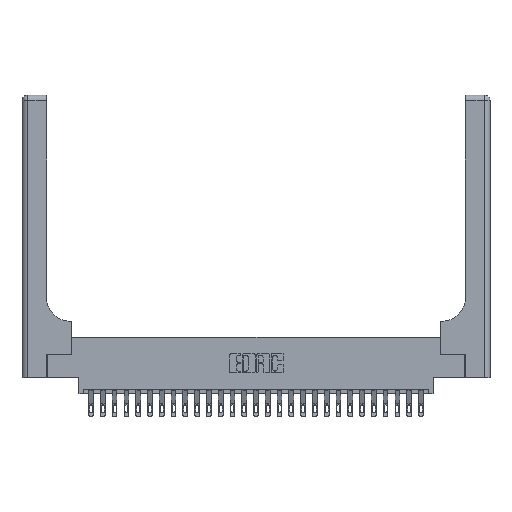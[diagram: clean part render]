
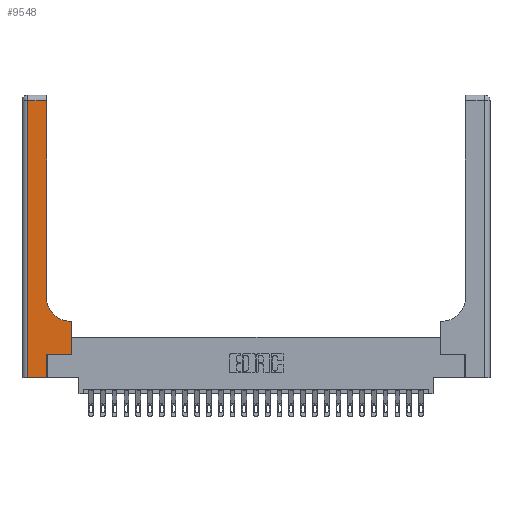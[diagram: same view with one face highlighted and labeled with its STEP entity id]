
A CAD part, top view. The second image highlights one B-rep face of the part: STEP entity #9548.
In plain terms, the highlighted planar face has unit normal (0, 0, 1).
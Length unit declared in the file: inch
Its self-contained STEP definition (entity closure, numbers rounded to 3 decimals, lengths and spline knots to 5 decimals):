
#1039 = ORIENTED_EDGE ( 'NONE', *, *, #16703, .T. ) ;
#1097 = VERTEX_POINT ( 'NONE', #2122 ) ;
#1189 = DIRECTION ( 'NONE',  ( 1., 0., 0. ) ) ;
#1203 = DIRECTION ( 'NONE',  ( 0., 1., 0. ) ) ;
#1382 = CARTESIAN_POINT ( 'NONE',  ( 0.06, 2.94, 0.37 ) ) ;
#2122 = CARTESIAN_POINT ( 'NONE',  ( 0.528, 0.25, 0.37 ) ) ;
#2577 = ORIENTED_EDGE ( 'NONE', *, *, #18024, .T. ) ;
#2879 = VERTEX_POINT ( 'NONE', #22804 ) ;
#2985 = ORIENTED_EDGE ( 'NONE', *, *, #6645, .T. ) ;
#3223 = DIRECTION ( 'NONE',  ( 0., -1., 0. ) ) ;
#3308 = VECTOR ( 'NONE', #7425, 39.37008 ) ;
#3347 = DIRECTION ( 'NONE',  ( 0., 1., 0. ) ) ;
#3357 = EDGE_CURVE ( 'NONE', #15722, #1097, #18580, .T. ) ;
#3717 = FACE_OUTER_BOUND ( 'NONE', #11040, .T. ) ;
#3836 = EDGE_CURVE ( 'NONE', #4402, #20982, #22188, .T. ) ;
#4402 = VERTEX_POINT ( 'NONE', #9415 ) ;
#4758 = LINE ( 'NONE', #11741, #18013 ) ;
#5121 = CARTESIAN_POINT ( 'NONE',  ( 0.26, 3., 0.37 ) ) ;
#5827 = CARTESIAN_POINT ( 'NONE',  ( 0.26, 0.6, 0.37 ) ) ;
#6161 = CARTESIAN_POINT ( 'NONE',  ( 0., 3., 0.37 ) ) ;
#6615 = EDGE_CURVE ( 'NONE', #1097, #4402, #4758, .T. ) ;
#6645 = EDGE_CURVE ( 'NONE', #7899, #23184, #26251, .T. ) ;
#6893 = AXIS2_PLACEMENT_3D ( 'NONE', #6161, #26481, #7634 ) ;
#6977 = CARTESIAN_POINT ( 'NONE',  ( 0.26, 0.85, 0.37 ) ) ;
#7020 = ORIENTED_EDGE ( 'NONE', *, *, #3357, .T. ) ;
#7138 = VECTOR ( 'NONE', #3223, 39.37008 ) ;
#7425 = DIRECTION ( 'NONE',  ( -1., 0., 0. ) ) ;
#7537 = EDGE_CURVE ( 'NONE', #20982, #13207, #10696, .T. ) ;
#7634 = DIRECTION ( 'NONE',  ( -1., 0., 0. ) ) ;
#7815 = VECTOR ( 'NONE', #15946, 39.37008 ) ;
#7899 = VERTEX_POINT ( 'NONE', #11426 ) ;
#8038 = DIRECTION ( 'NONE',  ( 0., 1., 0. ) ) ;
#8981 = AXIS2_PLACEMENT_3D ( 'NONE', #17418, #17280, #1189 ) ;
#9383 = ORIENTED_EDGE ( 'NONE', *, *, #6615, .T. ) ;
#9415 = CARTESIAN_POINT ( 'NONE',  ( 0.528, 0.6, 0.37 ) ) ;
#9548 = ADVANCED_FACE ( 'NONE', ( #3717 ), #24299, .F. ) ;
#10696 = CIRCLE ( 'NONE', #8981, 0.25 ) ;
#10886 = ORIENTED_EDGE ( 'NONE', *, *, #20495, .T. ) ;
#11040 = EDGE_LOOP ( 'NONE', ( #1039, #2985, #2577, #16382, #10886, #7020, #9383, #20888, #12377 ) ) ;
#11426 = CARTESIAN_POINT ( 'NONE',  ( 0.26, 2.94, 0.37 ) ) ;
#11454 = EDGE_CURVE ( 'NONE', #12512, #2879, #13920, .T. ) ;
#11741 = CARTESIAN_POINT ( 'NONE',  ( 0.528, 0.25, 0.37 ) ) ;
#12377 = ORIENTED_EDGE ( 'NONE', *, *, #7537, .T. ) ;
#12512 = VERTEX_POINT ( 'NONE', #14476 ) ;
#12771 = CARTESIAN_POINT ( 'NONE',  ( 0.265, 0.25, 0.37 ) ) ;
#13207 = VERTEX_POINT ( 'NONE', #6977 ) ;
#13920 = LINE ( 'NONE', #20284, #7815 ) ;
#14476 = CARTESIAN_POINT ( 'NONE',  ( 0.06, 0., 0.37 ) ) ;
#15722 = VERTEX_POINT ( 'NONE', #12771 ) ;
#15927 = LINE ( 'NONE', #24207, #7138 ) ;
#15946 = DIRECTION ( 'NONE',  ( 1., 0., 0. ) ) ;
#16382 = ORIENTED_EDGE ( 'NONE', *, *, #11454, .T. ) ;
#16553 = CARTESIAN_POINT ( 'NONE',  ( 0.265, 0., 0.37 ) ) ;
#16668 = CARTESIAN_POINT ( 'NONE',  ( 0.265, 0.25, 0.37 ) ) ;
#16703 = EDGE_CURVE ( 'NONE', #13207, #7899, #26126, .T. ) ;
#17250 = VECTOR ( 'NONE', #20161, 39.37008 ) ;
#17280 = DIRECTION ( 'NONE',  ( 0., 0., -1. ) ) ;
#17418 = CARTESIAN_POINT ( 'NONE',  ( 0.51, 0.85, 0.37 ) ) ;
#18013 = VECTOR ( 'NONE', #3347, 39.37008 ) ;
#18024 = EDGE_CURVE ( 'NONE', #23184, #12512, #15927, .T. ) ;
#18580 = LINE ( 'NONE', #16668, #24404 ) ;
#20161 = DIRECTION ( 'NONE',  ( -1., 0., 0. ) ) ;
#20220 = VECTOR ( 'NONE', #8038, 39.37008 ) ;
#20284 = CARTESIAN_POINT ( 'NONE',  ( 0., 0., 0.37 ) ) ;
#20485 = LINE ( 'NONE', #16553, #20220 ) ;
#20495 = EDGE_CURVE ( 'NONE', #2879, #15722, #20485, .T. ) ;
#20888 = ORIENTED_EDGE ( 'NONE', *, *, #3836, .T. ) ;
#20982 = VERTEX_POINT ( 'NONE', #21466 ) ;
#21466 = CARTESIAN_POINT ( 'NONE',  ( 0.51, 0.6, 0.37 ) ) ;
#22188 = LINE ( 'NONE', #5827, #17250 ) ;
#22804 = CARTESIAN_POINT ( 'NONE',  ( 0.265, 0., 0.37 ) ) ;
#23184 = VERTEX_POINT ( 'NONE', #1382 ) ;
#23929 = VECTOR ( 'NONE', #1203, 39.37008 ) ;
#24207 = CARTESIAN_POINT ( 'NONE',  ( 0.06, 3., 0.37 ) ) ;
#24299 = PLANE ( 'NONE',  #6893 ) ;
#24404 = VECTOR ( 'NONE', #24946, 39.37008 ) ;
#24946 = DIRECTION ( 'NONE',  ( 1., 0., 0. ) ) ;
#25996 = CARTESIAN_POINT ( 'NONE',  ( 0., 2.94, 0.37 ) ) ;
#26126 = LINE ( 'NONE', #5121, #23929 ) ;
#26251 = LINE ( 'NONE', #25996, #3308 ) ;
#26481 = DIRECTION ( 'NONE',  ( 0., 0., -1. ) ) ;
